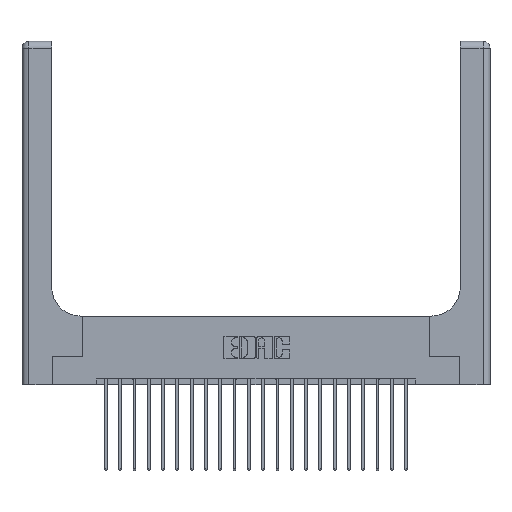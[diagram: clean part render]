
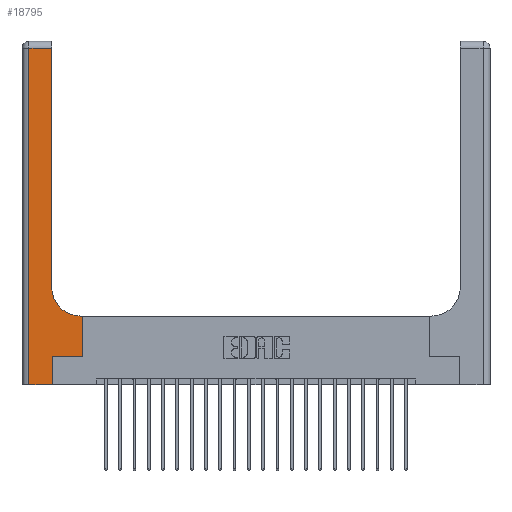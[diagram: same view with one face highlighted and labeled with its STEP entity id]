
A CAD part, top view. The second image highlights one B-rep face of the part: STEP entity #18795.
In plain terms, the highlighted planar face has unit normal (0, 0, 1).
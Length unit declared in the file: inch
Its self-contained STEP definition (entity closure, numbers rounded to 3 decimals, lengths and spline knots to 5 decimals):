
#112 = FACE_OUTER_BOUND ( 'NONE', #6702, .T. ) ;
#124 = CARTESIAN_POINT ( 'NONE',  ( 0.26, 0.85, 0.37 ) ) ;
#137 = ORIENTED_EDGE ( 'NONE', *, *, #3363, .T. ) ;
#260 = VECTOR ( 'NONE', #10446, 39.37008 ) ;
#543 = LINE ( 'NONE', #5820, #4586 ) ;
#1938 = DIRECTION ( 'NONE',  ( 0., 0., -1. ) ) ;
#2249 = EDGE_CURVE ( 'NONE', #8152, #20654, #11753, .T. ) ;
#2731 = ORIENTED_EDGE ( 'NONE', *, *, #4026, .T. ) ;
#2938 = ORIENTED_EDGE ( 'NONE', *, *, #2249, .T. ) ;
#3045 = LINE ( 'NONE', #4991, #13106 ) ;
#3132 = VERTEX_POINT ( 'NONE', #20997 ) ;
#3363 = EDGE_CURVE ( 'NONE', #21340, #8152, #543, .T. ) ;
#3577 = LINE ( 'NONE', #17601, #260 ) ;
#3592 = VECTOR ( 'NONE', #17114, 39.37008 ) ;
#3862 = AXIS2_PLACEMENT_3D ( 'NONE', #22424, #8274, #22099 ) ;
#4026 = EDGE_CURVE ( 'NONE', #12129, #12889, #13439, .T. ) ;
#4586 = VECTOR ( 'NONE', #14753, 39.37008 ) ;
#4900 = EDGE_CURVE ( 'NONE', #10187, #17272, #12439, .T. ) ;
#4991 = CARTESIAN_POINT ( 'NONE',  ( 0.26, 0.6, 0.37 ) ) ;
#5359 = EDGE_CURVE ( 'NONE', #3132, #10187, #3577, .T. ) ;
#5493 = ORIENTED_EDGE ( 'NONE', *, *, #20803, .T. ) ;
#5502 = CARTESIAN_POINT ( 'NONE',  ( 0.265, 0., 0.37 ) ) ;
#5820 = CARTESIAN_POINT ( 'NONE',  ( 0.06, 3., 0.37 ) ) ;
#6702 = EDGE_LOOP ( 'NONE', ( #10432, #9475, #137, #2938, #8332, #21062, #20014, #5493, #2731 ) ) ;
#7104 = PLANE ( 'NONE',  #12710 ) ;
#7420 = EDGE_CURVE ( 'NONE', #12889, #11931, #10054, .T. ) ;
#7634 = VECTOR ( 'NONE', #9124, 39.37008 ) ;
#8152 = VERTEX_POINT ( 'NONE', #11038 ) ;
#8274 = DIRECTION ( 'NONE',  ( 0., 0., -1. ) ) ;
#8332 = ORIENTED_EDGE ( 'NONE', *, *, #18697, .T. ) ;
#8366 = LINE ( 'NONE', #5502, #20824 ) ;
#8485 = LINE ( 'NONE', #15030, #3592 ) ;
#8948 = DIRECTION ( 'NONE',  ( -1., 0., 0. ) ) ;
#9124 = DIRECTION ( 'NONE',  ( 0., 1., 0. ) ) ;
#9233 = CARTESIAN_POINT ( 'NONE',  ( 0.528, 0.25, 0.37 ) ) ;
#9475 = ORIENTED_EDGE ( 'NONE', *, *, #20248, .T. ) ;
#10054 = LINE ( 'NONE', #11773, #21534 ) ;
#10187 = VERTEX_POINT ( 'NONE', #19685 ) ;
#10432 = ORIENTED_EDGE ( 'NONE', *, *, #7420, .T. ) ;
#10446 = DIRECTION ( 'NONE',  ( 1., 0., 0. ) ) ;
#10666 = CARTESIAN_POINT ( 'NONE',  ( 0., 3., 0.37 ) ) ;
#11038 = CARTESIAN_POINT ( 'NONE',  ( 0.06, 0., 0.37 ) ) ;
#11458 = CARTESIAN_POINT ( 'NONE',  ( 0.26, 2.94, 0.37 ) ) ;
#11647 = CARTESIAN_POINT ( 'NONE',  ( 0., 0., 0.37 ) ) ;
#11753 = LINE ( 'NONE', #11647, #22146 ) ;
#11773 = CARTESIAN_POINT ( 'NONE',  ( 0.26, 3., 0.37 ) ) ;
#11931 = VERTEX_POINT ( 'NONE', #11458 ) ;
#12129 = VERTEX_POINT ( 'NONE', #12587 ) ;
#12439 = LINE ( 'NONE', #9233, #7634 ) ;
#12465 = CARTESIAN_POINT ( 'NONE',  ( 0.06, 2.94, 0.37 ) ) ;
#12587 = CARTESIAN_POINT ( 'NONE',  ( 0.51, 0.6, 0.37 ) ) ;
#12710 = AXIS2_PLACEMENT_3D ( 'NONE', #10666, #1938, #8948 ) ;
#12889 = VERTEX_POINT ( 'NONE', #124 ) ;
#13106 = VECTOR ( 'NONE', #15320, 39.37008 ) ;
#13439 = CIRCLE ( 'NONE', #3862, 0.25 ) ;
#14154 = CARTESIAN_POINT ( 'NONE',  ( 0.528, 0.6, 0.37 ) ) ;
#14753 = DIRECTION ( 'NONE',  ( 0., -1., 0. ) ) ;
#15030 = CARTESIAN_POINT ( 'NONE',  ( 0., 2.94, 0.37 ) ) ;
#15320 = DIRECTION ( 'NONE',  ( -1., 0., 0. ) ) ;
#15321 = DIRECTION ( 'NONE',  ( 0., 1., 0. ) ) ;
#17114 = DIRECTION ( 'NONE',  ( -1., 0., 0. ) ) ;
#17272 = VERTEX_POINT ( 'NONE', #14154 ) ;
#17601 = CARTESIAN_POINT ( 'NONE',  ( 0.265, 0.25, 0.37 ) ) ;
#18697 = EDGE_CURVE ( 'NONE', #20654, #3132, #8366, .T. ) ;
#18795 = ADVANCED_FACE ( 'NONE', ( #112 ), #7104, .F. ) ;
#19685 = CARTESIAN_POINT ( 'NONE',  ( 0.528, 0.25, 0.37 ) ) ;
#19981 = CARTESIAN_POINT ( 'NONE',  ( 0.265, 0., 0.37 ) ) ;
#20014 = ORIENTED_EDGE ( 'NONE', *, *, #4900, .T. ) ;
#20248 = EDGE_CURVE ( 'NONE', #11931, #21340, #8485, .T. ) ;
#20654 = VERTEX_POINT ( 'NONE', #19981 ) ;
#20803 = EDGE_CURVE ( 'NONE', #17272, #12129, #3045, .T. ) ;
#20824 = VECTOR ( 'NONE', #21267, 39.37008 ) ;
#20997 = CARTESIAN_POINT ( 'NONE',  ( 0.265, 0.25, 0.37 ) ) ;
#21062 = ORIENTED_EDGE ( 'NONE', *, *, #5359, .T. ) ;
#21267 = DIRECTION ( 'NONE',  ( 0., 1., 0. ) ) ;
#21340 = VERTEX_POINT ( 'NONE', #12465 ) ;
#21534 = VECTOR ( 'NONE', #15321, 39.37008 ) ;
#22099 = DIRECTION ( 'NONE',  ( 1., 0., 0. ) ) ;
#22120 = DIRECTION ( 'NONE',  ( 1., 0., 0. ) ) ;
#22146 = VECTOR ( 'NONE', #22120, 39.37008 ) ;
#22424 = CARTESIAN_POINT ( 'NONE',  ( 0.51, 0.85, 0.37 ) ) ;
